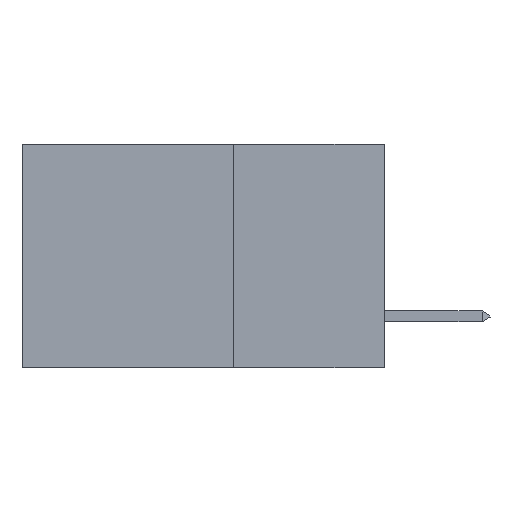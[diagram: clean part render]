
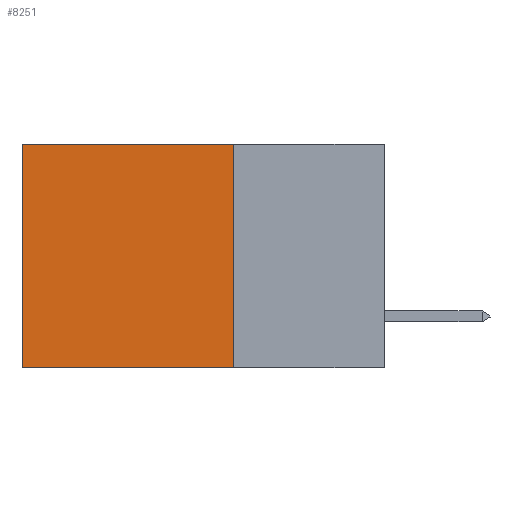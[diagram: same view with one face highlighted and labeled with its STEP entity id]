
A CAD part, left-side view. The second image highlights one B-rep face of the part: STEP entity #8251.
In plain terms, the highlighted planar face has unit normal (-1, 0, 0).
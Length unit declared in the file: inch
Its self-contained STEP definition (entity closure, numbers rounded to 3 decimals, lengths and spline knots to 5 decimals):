
#712 = VERTEX_POINT ( 'NONE', #8829 ) ;
#740 = ORIENTED_EDGE ( 'NONE', *, *, #3264, .F. ) ;
#1391 = CARTESIAN_POINT ( 'NONE',  ( 0.2875, 0.6, 0. ) ) ;
#2349 = LINE ( 'NONE', #3970, #2877 ) ;
#2646 = DIRECTION ( 'NONE',  ( 0., 0., -1. ) ) ;
#2676 = DIRECTION ( 'NONE',  ( 0., 1., 0. ) ) ;
#2877 = VECTOR ( 'NONE', #2646, 39.37008 ) ;
#2942 = DIRECTION ( 'NONE',  ( 0., 1., 0. ) ) ;
#3264 = EDGE_CURVE ( 'NONE', #15052, #13475, #15553, .T. ) ;
#3523 = CARTESIAN_POINT ( 'NONE',  ( 0.2875, 0.25, 0. ) ) ;
#3970 = CARTESIAN_POINT ( 'NONE',  ( 0.2875, 0.6, 0. ) ) ;
#4364 = FACE_OUTER_BOUND ( 'NONE', #10934, .T. ) ;
#5050 = PLANE ( 'NONE',  #7910 ) ;
#6142 = EDGE_CURVE ( 'NONE', #8713, #712, #2349, .T. ) ;
#6976 = LINE ( 'NONE', #14466, #13017 ) ;
#7302 = DIRECTION ( 'NONE',  ( 0., 0., -1. ) ) ;
#7910 = AXIS2_PLACEMENT_3D ( 'NONE', #3523, #18681, #15028 ) ;
#8251 = ADVANCED_FACE ( 'NONE', ( #4364 ), #5050, .F. ) ;
#8713 = VERTEX_POINT ( 'NONE', #1391 ) ;
#8829 = CARTESIAN_POINT ( 'NONE',  ( 0.2875, 0.6, -0.37 ) ) ;
#10687 = EDGE_CURVE ( 'NONE', #13475, #712, #6976, .T. ) ;
#10772 = CARTESIAN_POINT ( 'NONE',  ( 0.2875, 0.25, 0. ) ) ;
#10812 = ORIENTED_EDGE ( 'NONE', *, *, #10687, .F. ) ;
#10934 = EDGE_LOOP ( 'NONE', ( #13104, #10812, #740, #11483 ) ) ;
#11483 = ORIENTED_EDGE ( 'NONE', *, *, #11946, .T. ) ;
#11946 = EDGE_CURVE ( 'NONE', #15052, #8713, #18926, .T. ) ;
#13017 = VECTOR ( 'NONE', #2942, 39.37008 ) ;
#13104 = ORIENTED_EDGE ( 'NONE', *, *, #6142, .T. ) ;
#13475 = VERTEX_POINT ( 'NONE', #14987 ) ;
#14403 = CARTESIAN_POINT ( 'NONE',  ( 0.2875, 0.25, 0. ) ) ;
#14466 = CARTESIAN_POINT ( 'NONE',  ( 0.2875, 0.25, -0.37 ) ) ;
#14987 = CARTESIAN_POINT ( 'NONE',  ( 0.2875, 0.25, -0.37 ) ) ;
#15028 = DIRECTION ( 'NONE',  ( 0., 0., -1. ) ) ;
#15052 = VERTEX_POINT ( 'NONE', #15708 ) ;
#15553 = LINE ( 'NONE', #10772, #20535 ) ;
#15708 = CARTESIAN_POINT ( 'NONE',  ( 0.2875, 0.25, 0. ) ) ;
#18681 = DIRECTION ( 'NONE',  ( 1., 0., 0. ) ) ;
#18926 = LINE ( 'NONE', #14403, #20503 ) ;
#20503 = VECTOR ( 'NONE', #2676, 39.37008 ) ;
#20535 = VECTOR ( 'NONE', #7302, 39.37008 ) ;
